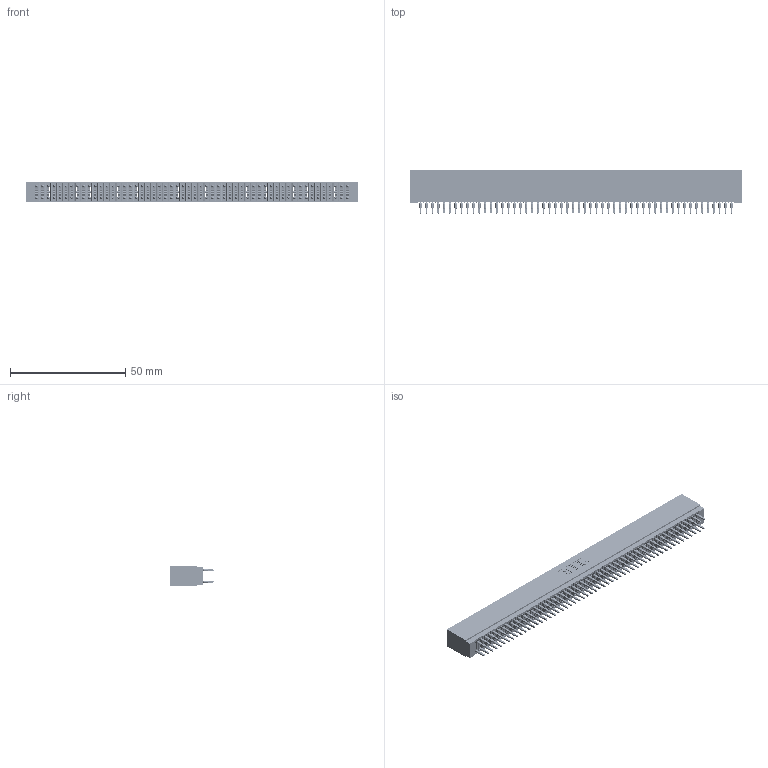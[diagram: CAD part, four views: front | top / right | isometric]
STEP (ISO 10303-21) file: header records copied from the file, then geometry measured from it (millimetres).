
FILE_DESCRIPTION (( 'STEP AP203' ), '1' );
FILE_NAME ('725-108-560-201.STEP', '2026-02-24T20:25:38', ( '' ), ( '' ), 'SwSTEP 2.0', 'SolidWorks 2023', '' );
FILE_SCHEMA (( 'CONFIG_CONTROL_DESIGN' ));
Length unit declared in the file: millimetre
Products named in the file (3): 725-108-560-201; 745-292-001_560; 725 Part_Insulator Option - 01
Assembly tree (109 placements, depth 2):
  725-108-560-201
    725 Part_Insulator Option - 01
    745-292-001_560  x108
Bounding box: 143.76 x 18.8 x 8.89 mm (x, y, z)
Volume: 11739.1 mm3; surface area: 26754.1 mm2
Topology: 109 solids, 109 shells, 10733 faces, 29360 edges, 18636 vertices
Faces by surface type: plane 5563, cylinder 2362, bspline 2160, torus 648
Entity records: 89559 total; most frequent: CARTESIAN_POINT 16033, ORIENTED_EDGE 15492, DIRECTION 13530, EDGE_CURVE 7746, VECTOR 7232, LINE 7232, VERTEX_POINT 4940, AXIS2_PLACEMENT_3D 3149
